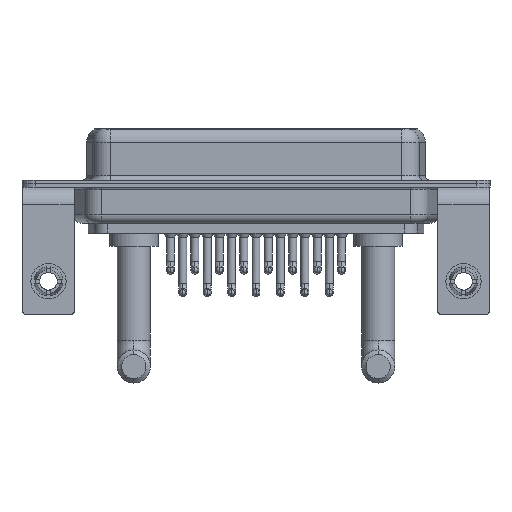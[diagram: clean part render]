
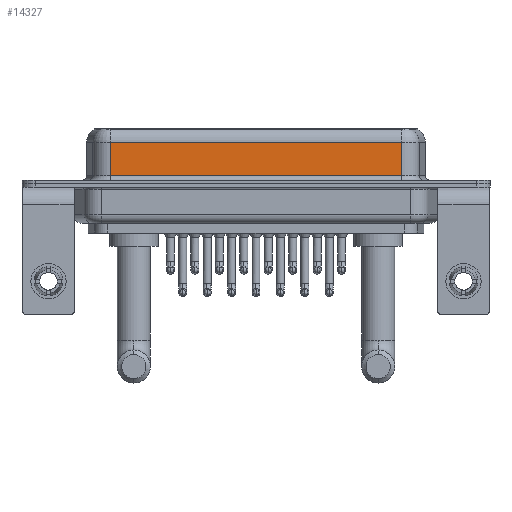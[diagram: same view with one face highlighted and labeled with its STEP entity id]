
A CAD part, front view. The second image highlights one B-rep face of the part: STEP entity #14327.
In plain terms, the highlighted planar face has unit normal (0, -1, 0).
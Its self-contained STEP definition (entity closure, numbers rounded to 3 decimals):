
#268 = CARTESIAN_POINT ( 'NONE',  ( 40.037, -3.95, 0.9 ) ) ;
#711 = CARTESIAN_POINT ( 'NONE',  ( 7.013, -3.95, 0.9 ) ) ;
#756 = FACE_OUTER_BOUND ( 'NONE', #11942, .T. ) ;
#801 = VECTOR ( 'NONE', #17270, 1000. ) ;
#1236 = EDGE_CURVE ( 'NONE', #7361, #3439, #9704, .T. ) ;
#1530 = CARTESIAN_POINT ( 'NONE',  ( 40.037, -3.95, 6.4 ) ) ;
#1897 = ORIENTED_EDGE ( 'NONE', *, *, #13719, .F. ) ;
#2051 = CARTESIAN_POINT ( 'NONE',  ( 7.013, -3.95, 6.4 ) ) ;
#2401 = DIRECTION ( 'NONE',  ( 0., 0., 1. ) ) ;
#2466 = ORIENTED_EDGE ( 'NONE', *, *, #11857, .T. ) ;
#3080 = LINE ( 'NONE', #1530, #20011 ) ;
#3439 = VERTEX_POINT ( 'NONE', #268 ) ;
#4301 = DIRECTION ( 'NONE',  ( 1., 0., 0. ) ) ;
#5895 = VECTOR ( 'NONE', #9224, 1000. ) ;
#6698 = CARTESIAN_POINT ( 'NONE',  ( 7.013, -3.95, 4.65 ) ) ;
#6712 = DIRECTION ( 'NONE',  ( 0., 0., -1. ) ) ;
#7361 = VERTEX_POINT ( 'NONE', #711 ) ;
#7492 = CARTESIAN_POINT ( 'NONE',  ( 40.037, -3.95, 0.9 ) ) ;
#7810 = PLANE ( 'NONE',  #11775 ) ;
#9224 = DIRECTION ( 'NONE',  ( 0., 0., -1. ) ) ;
#9589 = CARTESIAN_POINT ( 'NONE',  ( 40.037, -3.95, 4.65 ) ) ;
#9697 = ORIENTED_EDGE ( 'NONE', *, *, #1236, .T. ) ;
#9704 = LINE ( 'NONE', #7492, #22328 ) ;
#10330 = CARTESIAN_POINT ( 'NONE',  ( 40.037, -3.95, 4.65 ) ) ;
#10674 = VERTEX_POINT ( 'NONE', #9589 ) ;
#11775 = AXIS2_PLACEMENT_3D ( 'NONE', #16636, #18287, #2401 ) ;
#11857 = EDGE_CURVE ( 'NONE', #21190, #7361, #12736, .T. ) ;
#11942 = EDGE_LOOP ( 'NONE', ( #1897, #23003, #2466, #9697 ) ) ;
#12736 = LINE ( 'NONE', #2051, #5895 ) ;
#13719 = EDGE_CURVE ( 'NONE', #10674, #3439, #3080, .T. ) ;
#14327 = ADVANCED_FACE ( 'NONE', ( #756 ), #7810, .F. ) ;
#16636 = CARTESIAN_POINT ( 'NONE',  ( 40.037, -3.95, 6.4 ) ) ;
#17270 = DIRECTION ( 'NONE',  ( -1., 0., 0. ) ) ;
#18015 = EDGE_CURVE ( 'NONE', #10674, #21190, #22800, .T. ) ;
#18287 = DIRECTION ( 'NONE',  ( 0., 1., 0. ) ) ;
#20011 = VECTOR ( 'NONE', #6712, 1000. ) ;
#21190 = VERTEX_POINT ( 'NONE', #6698 ) ;
#22328 = VECTOR ( 'NONE', #4301, 1000. ) ;
#22800 = LINE ( 'NONE', #10330, #801 ) ;
#23003 = ORIENTED_EDGE ( 'NONE', *, *, #18015, .T. ) ;
